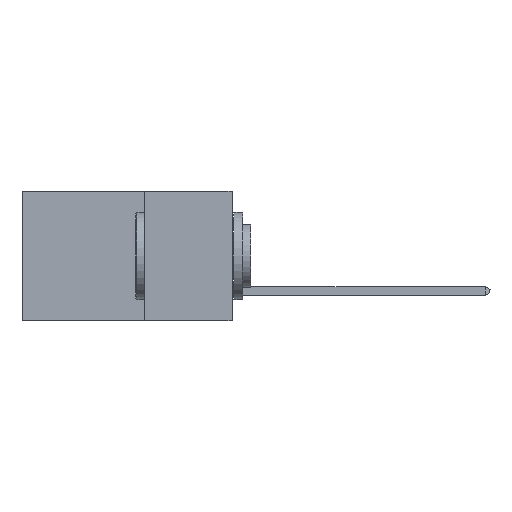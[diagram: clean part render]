
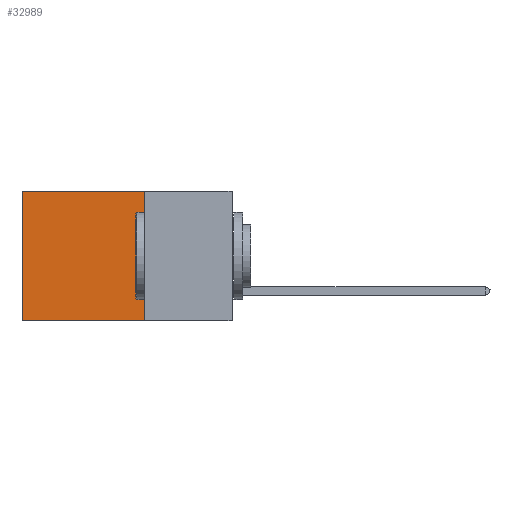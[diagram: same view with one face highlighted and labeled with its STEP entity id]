
A CAD part, left-side view. The second image highlights one B-rep face of the part: STEP entity #32989.
In plain terms, the highlighted planar face has unit normal (-1, 0, 0).
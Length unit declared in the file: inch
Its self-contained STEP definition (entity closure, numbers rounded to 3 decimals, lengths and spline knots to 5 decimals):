
#2296 = ORIENTED_EDGE ( 'NONE', *, *, #38003, .F. ) ;
#4860 = VERTEX_POINT ( 'NONE', #17805 ) ;
#5255 = VERTEX_POINT ( 'NONE', #8821 ) ;
#6219 = ORIENTED_EDGE ( 'NONE', *, *, #37115, .F. ) ;
#6809 = DIRECTION ( 'NONE',  ( 0., 0., -1. ) ) ;
#7888 = CARTESIAN_POINT ( 'NONE',  ( 0.2875, 0.25, 0. ) ) ;
#8644 = LINE ( 'NONE', #32408, #34248 ) ;
#8821 = CARTESIAN_POINT ( 'NONE',  ( 0.2875, 0.6, 0. ) ) ;
#9043 = LINE ( 'NONE', #25641, #30291 ) ;
#10345 = DIRECTION ( 'NONE',  ( 1., 0., 0. ) ) ;
#13312 = PLANE ( 'NONE',  #28938 ) ;
#14242 = EDGE_LOOP ( 'NONE', ( #28665, #6219, #2296, #22118 ) ) ;
#16474 = CARTESIAN_POINT ( 'NONE',  ( 0.2875, 0.25, 0. ) ) ;
#16612 = DIRECTION ( 'NONE',  ( 0., 0., -1. ) ) ;
#16903 = VECTOR ( 'NONE', #35037, 39.37008 ) ;
#17195 = EDGE_CURVE ( 'NONE', #34728, #5255, #23203, .T. ) ;
#17805 = CARTESIAN_POINT ( 'NONE',  ( 0.2875, 0.6, -0.37 ) ) ;
#18731 = CARTESIAN_POINT ( 'NONE',  ( 0.2875, 0.25, -0.37 ) ) ;
#19531 = CARTESIAN_POINT ( 'NONE',  ( 0.2875, 0.6, 0. ) ) ;
#19832 = EDGE_CURVE ( 'NONE', #5255, #4860, #29663, .T. ) ;
#21523 = VECTOR ( 'NONE', #22511, 39.37008 ) ;
#22118 = ORIENTED_EDGE ( 'NONE', *, *, #17195, .T. ) ;
#22511 = DIRECTION ( 'NONE',  ( 0., 0., -1. ) ) ;
#23203 = LINE ( 'NONE', #34898, #16903 ) ;
#23794 = VERTEX_POINT ( 'NONE', #18731 ) ;
#25641 = CARTESIAN_POINT ( 'NONE',  ( 0.2875, 0.25, 0. ) ) ;
#26239 = DIRECTION ( 'NONE',  ( 0., 1., 0. ) ) ;
#27475 = FACE_OUTER_BOUND ( 'NONE', #14242, .T. ) ;
#28665 = ORIENTED_EDGE ( 'NONE', *, *, #19832, .T. ) ;
#28938 = AXIS2_PLACEMENT_3D ( 'NONE', #16474, #10345, #16612 ) ;
#29663 = LINE ( 'NONE', #19531, #21523 ) ;
#30291 = VECTOR ( 'NONE', #6809, 39.37008 ) ;
#32408 = CARTESIAN_POINT ( 'NONE',  ( 0.2875, 0.25, -0.37 ) ) ;
#32989 = ADVANCED_FACE ( 'NONE', ( #27475 ), #13312, .F. ) ;
#34248 = VECTOR ( 'NONE', #26239, 39.37008 ) ;
#34728 = VERTEX_POINT ( 'NONE', #7888 ) ;
#34898 = CARTESIAN_POINT ( 'NONE',  ( 0.2875, 0.25, 0. ) ) ;
#35037 = DIRECTION ( 'NONE',  ( 0., 1., 0. ) ) ;
#37115 = EDGE_CURVE ( 'NONE', #23794, #4860, #8644, .T. ) ;
#38003 = EDGE_CURVE ( 'NONE', #34728, #23794, #9043, .T. ) ;
